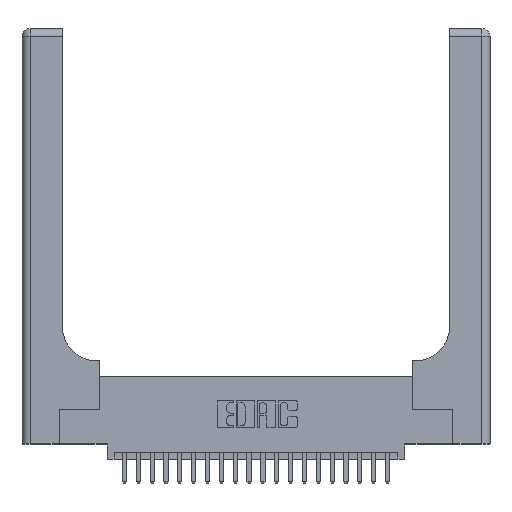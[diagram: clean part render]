
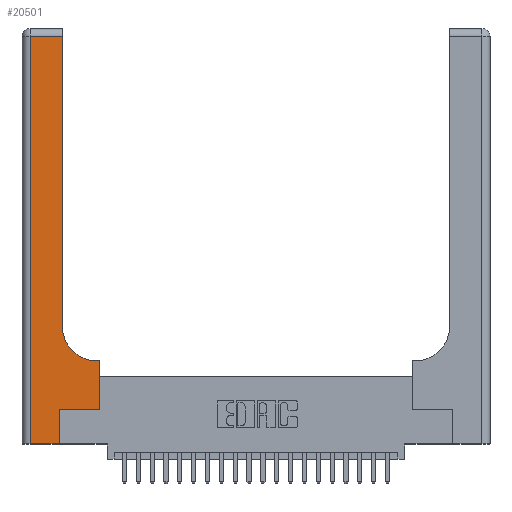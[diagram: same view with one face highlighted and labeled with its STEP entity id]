
A CAD part, top view. The second image highlights one B-rep face of the part: STEP entity #20501.
In plain terms, the highlighted planar face has unit normal (0, 0, 1).
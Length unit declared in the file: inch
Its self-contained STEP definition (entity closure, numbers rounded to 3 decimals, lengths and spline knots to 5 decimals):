
#212 = VECTOR ( 'NONE', #11050, 39.37008 ) ;
#438 = VERTEX_POINT ( 'NONE', #825 ) ;
#490 = ORIENTED_EDGE ( 'NONE', *, *, #5498, .T. ) ;
#815 = DIRECTION ( 'NONE',  ( 1., 0., 0. ) ) ;
#825 = CARTESIAN_POINT ( 'NONE',  ( 0.06, 0., 0.37 ) ) ;
#970 = VECTOR ( 'NONE', #17006, 39.37008 ) ;
#1034 = VERTEX_POINT ( 'NONE', #4964 ) ;
#1068 = VERTEX_POINT ( 'NONE', #13298 ) ;
#1161 = DIRECTION ( 'NONE',  ( 0., 0., -1. ) ) ;
#1691 = CARTESIAN_POINT ( 'NONE',  ( 0.5585, 0.6, 0.37 ) ) ;
#1879 = EDGE_CURVE ( 'NONE', #11692, #1034, #5384, .T. ) ;
#1922 = EDGE_CURVE ( 'NONE', #16342, #14991, #19610, .T. ) ;
#2332 = DIRECTION ( 'NONE',  ( -1., 0., 0. ) ) ;
#3115 = FACE_OUTER_BOUND ( 'NONE', #16448, .T. ) ;
#3578 = VECTOR ( 'NONE', #815, 39.37008 ) ;
#3670 = CARTESIAN_POINT ( 'NONE',  ( 0.2915, 0.85, 0.37 ) ) ;
#3930 = CARTESIAN_POINT ( 'NONE',  ( 0.2915, 3., 0.37 ) ) ;
#4358 = AXIS2_PLACEMENT_3D ( 'NONE', #10689, #1161, #14378 ) ;
#4448 = ORIENTED_EDGE ( 'NONE', *, *, #1879, .T. ) ;
#4851 = LINE ( 'NONE', #18302, #14212 ) ;
#4964 = CARTESIAN_POINT ( 'NONE',  ( 0.5415, 0.6, 0.37 ) ) ;
#5249 = EDGE_CURVE ( 'NONE', #438, #16298, #8618, .T. ) ;
#5384 = LINE ( 'NONE', #11282, #212 ) ;
#5498 = EDGE_CURVE ( 'NONE', #16298, #16342, #13821, .T. ) ;
#5553 = VECTOR ( 'NONE', #18938, 39.37008 ) ;
#5951 = AXIS2_PLACEMENT_3D ( 'NONE', #21605, #10677, #23384 ) ;
#5987 = ORIENTED_EDGE ( 'NONE', *, *, #8935, .T. ) ;
#7945 = ORIENTED_EDGE ( 'NONE', *, *, #5249, .T. ) ;
#8618 = LINE ( 'NONE', #17678, #3578 ) ;
#8935 = EDGE_CURVE ( 'NONE', #11679, #1068, #23891, .T. ) ;
#9090 = ORIENTED_EDGE ( 'NONE', *, *, #14184, .T. ) ;
#9202 = DIRECTION ( 'NONE',  ( 0., 1., 0. ) ) ;
#9253 = VECTOR ( 'NONE', #10231, 39.37008 ) ;
#9893 = ORIENTED_EDGE ( 'NONE', *, *, #9926, .T. ) ;
#9926 = EDGE_CURVE ( 'NONE', #1034, #11679, #19085, .T. ) ;
#10158 = CARTESIAN_POINT ( 'NONE',  ( 0.269, 0.25, 0.37 ) ) ;
#10231 = DIRECTION ( 'NONE',  ( 1., 0., 0. ) ) ;
#10677 = DIRECTION ( 'NONE',  ( 0., 0., -1. ) ) ;
#10689 = CARTESIAN_POINT ( 'NONE',  ( 0., 3., 0.37 ) ) ;
#11050 = DIRECTION ( 'NONE',  ( -1., 0., 0. ) ) ;
#11282 = CARTESIAN_POINT ( 'NONE',  ( 0.2915, 0.6, 0.37 ) ) ;
#11679 = VERTEX_POINT ( 'NONE', #3670 ) ;
#11692 = VERTEX_POINT ( 'NONE', #1691 ) ;
#13298 = CARTESIAN_POINT ( 'NONE',  ( 0.2915, 2.94, 0.37 ) ) ;
#13578 = EDGE_CURVE ( 'NONE', #14991, #11692, #15489, .T. ) ;
#13821 = LINE ( 'NONE', #22004, #24022 ) ;
#14184 = EDGE_CURVE ( 'NONE', #1068, #19050, #18596, .T. ) ;
#14212 = VECTOR ( 'NONE', #21927, 39.37008 ) ;
#14378 = DIRECTION ( 'NONE',  ( -1., 0., 0. ) ) ;
#14991 = VERTEX_POINT ( 'NONE', #21259 ) ;
#15281 = CARTESIAN_POINT ( 'NONE',  ( 0.5585, 0.25, 0.37 ) ) ;
#15489 = LINE ( 'NONE', #15281, #5553 ) ;
#15948 = EDGE_CURVE ( 'NONE', #19050, #438, #4851, .T. ) ;
#16140 = ORIENTED_EDGE ( 'NONE', *, *, #1922, .T. ) ;
#16298 = VERTEX_POINT ( 'NONE', #19543 ) ;
#16342 = VERTEX_POINT ( 'NONE', #19704 ) ;
#16448 = EDGE_LOOP ( 'NONE', ( #5987, #9090, #22012, #7945, #490, #16140, #16765, #4448, #9893 ) ) ;
#16765 = ORIENTED_EDGE ( 'NONE', *, *, #13578, .T. ) ;
#17006 = DIRECTION ( 'NONE',  ( 0., 1., 0. ) ) ;
#17678 = CARTESIAN_POINT ( 'NONE',  ( 0., 0., 0.37 ) ) ;
#18302 = CARTESIAN_POINT ( 'NONE',  ( 0.06, 3., 0.37 ) ) ;
#18596 = LINE ( 'NONE', #18989, #21703 ) ;
#18938 = DIRECTION ( 'NONE',  ( 0., 1., 0. ) ) ;
#18989 = CARTESIAN_POINT ( 'NONE',  ( 0., 2.94, 0.37 ) ) ;
#19050 = VERTEX_POINT ( 'NONE', #21775 ) ;
#19085 = CIRCLE ( 'NONE', #5951, 0.25 ) ;
#19543 = CARTESIAN_POINT ( 'NONE',  ( 0.269, 0., 0.37 ) ) ;
#19610 = LINE ( 'NONE', #10158, #9253 ) ;
#19704 = CARTESIAN_POINT ( 'NONE',  ( 0.269, 0.25, 0.37 ) ) ;
#20501 = ADVANCED_FACE ( 'NONE', ( #3115 ), #23392, .F. ) ;
#21259 = CARTESIAN_POINT ( 'NONE',  ( 0.5585, 0.25, 0.37 ) ) ;
#21605 = CARTESIAN_POINT ( 'NONE',  ( 0.5415, 0.85, 0.37 ) ) ;
#21703 = VECTOR ( 'NONE', #2332, 39.37008 ) ;
#21775 = CARTESIAN_POINT ( 'NONE',  ( 0.06, 2.94, 0.37 ) ) ;
#21927 = DIRECTION ( 'NONE',  ( 0., -1., 0. ) ) ;
#22004 = CARTESIAN_POINT ( 'NONE',  ( 0.269, 0., 0.37 ) ) ;
#22012 = ORIENTED_EDGE ( 'NONE', *, *, #15948, .T. ) ;
#23384 = DIRECTION ( 'NONE',  ( 1., 0., 0. ) ) ;
#23392 = PLANE ( 'NONE',  #4358 ) ;
#23891 = LINE ( 'NONE', #3930, #970 ) ;
#24022 = VECTOR ( 'NONE', #9202, 39.37008 ) ;
